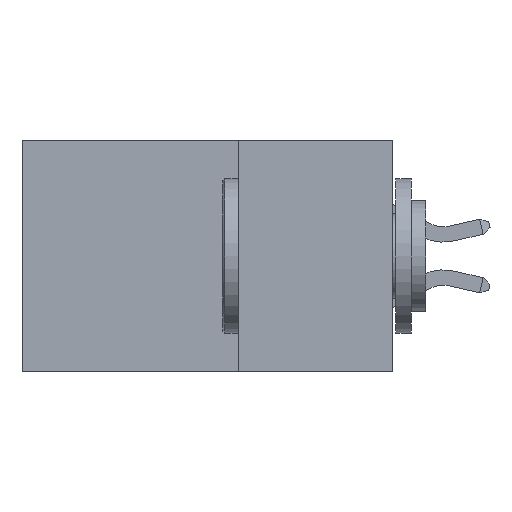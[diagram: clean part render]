
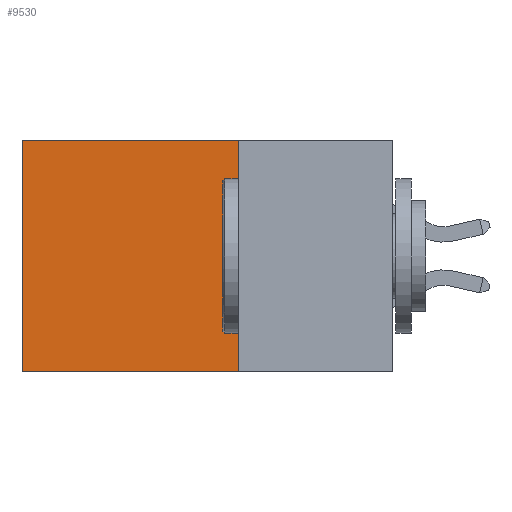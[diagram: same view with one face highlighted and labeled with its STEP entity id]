
A CAD part, left-side view. The second image highlights one B-rep face of the part: STEP entity #9530.
In plain terms, the highlighted planar face has unit normal (-1, 0, 0).
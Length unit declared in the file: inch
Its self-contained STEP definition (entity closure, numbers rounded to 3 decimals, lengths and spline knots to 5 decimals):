
#27 = CARTESIAN_POINT ( 'NONE',  ( 0.2875, 0.25, -0.375 ) ) ;
#1265 = EDGE_CURVE ( 'NONE', #4672, #11516, #9029, .T. ) ;
#1851 = EDGE_CURVE ( 'NONE', #7791, #15628, #13221, .T. ) ;
#2002 = CARTESIAN_POINT ( 'NONE',  ( 0.2875, 0.6, -0.375 ) ) ;
#2994 = LINE ( 'NONE', #10420, #13637 ) ;
#4108 = CARTESIAN_POINT ( 'NONE',  ( 0.2875, 0.6, 0. ) ) ;
#4672 = VERTEX_POINT ( 'NONE', #4108 ) ;
#5050 = DIRECTION ( 'NONE',  ( 1., 0., 0. ) ) ;
#5393 = DIRECTION ( 'NONE',  ( 0., 1., 0. ) ) ;
#5521 = FACE_OUTER_BOUND ( 'NONE', #11182, .T. ) ;
#6171 = VECTOR ( 'NONE', #6245, 39.37008 ) ;
#6245 = DIRECTION ( 'NONE',  ( 0., 0., -1. ) ) ;
#6398 = DIRECTION ( 'NONE',  ( 0., 0., -1. ) ) ;
#7675 = ORIENTED_EDGE ( 'NONE', *, *, #11155, .F. ) ;
#7791 = VERTEX_POINT ( 'NONE', #14719 ) ;
#7845 = DIRECTION ( 'NONE',  ( 0., 1., 0. ) ) ;
#8017 = DIRECTION ( 'NONE',  ( 0., 0., -1. ) ) ;
#8125 = LINE ( 'NONE', #10665, #11723 ) ;
#9029 = LINE ( 'NONE', #14136, #6171 ) ;
#9530 = ADVANCED_FACE ( 'NONE', ( #5521 ), #15278, .F. ) ;
#10420 = CARTESIAN_POINT ( 'NONE',  ( 0.2875, 0.25, 0. ) ) ;
#10546 = CARTESIAN_POINT ( 'NONE',  ( 0.2875, 0.25, -0.375 ) ) ;
#10665 = CARTESIAN_POINT ( 'NONE',  ( 0.2875, 0.25, -0.375 ) ) ;
#11155 = EDGE_CURVE ( 'NONE', #15628, #11516, #8125, .T. ) ;
#11182 = EDGE_LOOP ( 'NONE', ( #13016, #7675, #14984, #12358 ) ) ;
#11208 = VECTOR ( 'NONE', #8017, 39.37008 ) ;
#11516 = VERTEX_POINT ( 'NONE', #2002 ) ;
#11638 = CARTESIAN_POINT ( 'NONE',  ( 0.2875, 0.25, -0.375 ) ) ;
#11723 = VECTOR ( 'NONE', #7845, 39.37008 ) ;
#12358 = ORIENTED_EDGE ( 'NONE', *, *, #13521, .T. ) ;
#13016 = ORIENTED_EDGE ( 'NONE', *, *, #1265, .T. ) ;
#13221 = LINE ( 'NONE', #10546, #11208 ) ;
#13521 = EDGE_CURVE ( 'NONE', #7791, #4672, #2994, .T. ) ;
#13637 = VECTOR ( 'NONE', #5393, 39.37008 ) ;
#14136 = CARTESIAN_POINT ( 'NONE',  ( 0.2875, 0.6, -0.375 ) ) ;
#14719 = CARTESIAN_POINT ( 'NONE',  ( 0.2875, 0.25, 0. ) ) ;
#14984 = ORIENTED_EDGE ( 'NONE', *, *, #1851, .F. ) ;
#15278 = PLANE ( 'NONE',  #15472 ) ;
#15472 = AXIS2_PLACEMENT_3D ( 'NONE', #11638, #5050, #6398 ) ;
#15628 = VERTEX_POINT ( 'NONE', #27 ) ;
